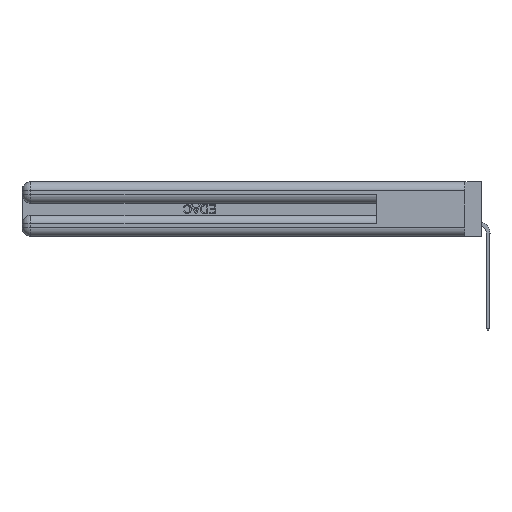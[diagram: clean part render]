
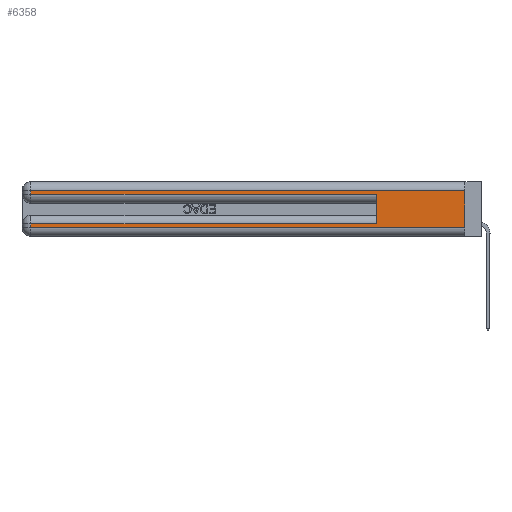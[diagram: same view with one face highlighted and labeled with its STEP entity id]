
A CAD part, left-side view. The second image highlights one B-rep face of the part: STEP entity #6358.
In plain terms, the highlighted planar face has unit normal (-1, 0, 0).
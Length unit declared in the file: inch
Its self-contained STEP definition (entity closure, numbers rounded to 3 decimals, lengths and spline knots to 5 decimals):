
#982 = ORIENTED_EDGE ( 'NONE', *, *, #1939, .T. ) ;
#1150 = CARTESIAN_POINT ( 'NONE',  ( 0., 0., 0.285 ) ) ;
#1248 = EDGE_CURVE ( 'NONE', #21710, #50398, #15956, .T. ) ;
#1607 = DIRECTION ( 'NONE',  ( 0., 0., 1. ) ) ;
#1939 = EDGE_CURVE ( 'NONE', #13976, #37767, #22024, .T. ) ;
#2253 = CARTESIAN_POINT ( 'NONE',  ( 0., 0., 0.37 ) ) ;
#3500 = ORIENTED_EDGE ( 'NONE', *, *, #37132, .T. ) ;
#4150 = VECTOR ( 'NONE', #22896, 39.37008 ) ;
#5775 = VECTOR ( 'NONE', #38353, 39.37008 ) ;
#6358 = ADVANCED_FACE ( 'NONE', ( #45294 ), #34544, .F. ) ;
#6715 = DIRECTION ( 'NONE',  ( 0., -1., 0. ) ) ;
#7668 = ORIENTED_EDGE ( 'NONE', *, *, #10380, .T. ) ;
#8444 = DIRECTION ( 'NONE',  ( 0., 1., 0. ) ) ;
#9440 = LINE ( 'NONE', #10826, #5775 ) ;
#9515 = CARTESIAN_POINT ( 'NONE',  ( 0., 2.94, 0.06 ) ) ;
#9645 = CARTESIAN_POINT ( 'NONE',  ( 0., 2.94, 0.37 ) ) ;
#10380 = EDGE_CURVE ( 'NONE', #46053, #13976, #9440, .T. ) ;
#10826 = CARTESIAN_POINT ( 'NONE',  ( 0., 2.94, 0.37 ) ) ;
#13364 = CARTESIAN_POINT ( 'NONE',  ( 0., 0.6, 0.145 ) ) ;
#13976 = VERTEX_POINT ( 'NONE', #9515 ) ;
#15003 = CARTESIAN_POINT ( 'NONE',  ( 0., 0., 0.085 ) ) ;
#15956 = LINE ( 'NONE', #13364, #32484 ) ;
#16480 = EDGE_CURVE ( 'NONE', #42474, #50621, #39028, .T. ) ;
#18364 = ORIENTED_EDGE ( 'NONE', *, *, #24891, .T. ) ;
#21710 = VERTEX_POINT ( 'NONE', #35023 ) ;
#22024 = LINE ( 'NONE', #45511, #50157 ) ;
#22172 = CARTESIAN_POINT ( 'NONE',  ( 0., 2.94, 0.085 ) ) ;
#22503 = LINE ( 'NONE', #15003, #4150 ) ;
#22896 = DIRECTION ( 'NONE',  ( 0., 1., 0. ) ) ;
#22976 = CARTESIAN_POINT ( 'NONE',  ( 0., 2.94, 0.285 ) ) ;
#24891 = EDGE_CURVE ( 'NONE', #31855, #50398, #48122, .T. ) ;
#26126 = DIRECTION ( 'NONE',  ( 0., 0., -1. ) ) ;
#26190 = ORIENTED_EDGE ( 'NONE', *, *, #38431, .T. ) ;
#27035 = LINE ( 'NONE', #2253, #39302 ) ;
#27101 = CARTESIAN_POINT ( 'NONE',  ( 0., 0., 0.06 ) ) ;
#29644 = VECTOR ( 'NONE', #32854, 39.37008 ) ;
#30046 = AXIS2_PLACEMENT_3D ( 'NONE', #38516, #38168, #45825 ) ;
#31814 = CARTESIAN_POINT ( 'NONE',  ( 0., 0., 0.31 ) ) ;
#31855 = VERTEX_POINT ( 'NONE', #22976 ) ;
#32065 = LINE ( 'NONE', #9645, #29644 ) ;
#32356 = CARTESIAN_POINT ( 'NONE',  ( 0., 2.94, 0.31 ) ) ;
#32364 = CARTESIAN_POINT ( 'NONE',  ( 0., 0., 0.31 ) ) ;
#32484 = VECTOR ( 'NONE', #1607, 39.37008 ) ;
#32854 = DIRECTION ( 'NONE',  ( 0., 0., -1. ) ) ;
#33517 = ORIENTED_EDGE ( 'NONE', *, *, #40971, .F. ) ;
#33825 = ORIENTED_EDGE ( 'NONE', *, *, #16480, .T. ) ;
#34544 = PLANE ( 'NONE',  #30046 ) ;
#35023 = CARTESIAN_POINT ( 'NONE',  ( 0., 0.6, 0.085 ) ) ;
#37132 = EDGE_CURVE ( 'NONE', #21710, #46053, #22503, .T. ) ;
#37767 = VERTEX_POINT ( 'NONE', #27101 ) ;
#37785 = VECTOR ( 'NONE', #40123, 39.37008 ) ;
#38168 = DIRECTION ( 'NONE',  ( 1., 0., 0. ) ) ;
#38353 = DIRECTION ( 'NONE',  ( 0., 0., -1. ) ) ;
#38431 = EDGE_CURVE ( 'NONE', #50621, #31855, #32065, .T. ) ;
#38516 = CARTESIAN_POINT ( 'NONE',  ( 0., 0., 0.37 ) ) ;
#39028 = LINE ( 'NONE', #31814, #48142 ) ;
#39302 = VECTOR ( 'NONE', #26126, 39.37008 ) ;
#40123 = DIRECTION ( 'NONE',  ( 0., -1., 0. ) ) ;
#40971 = EDGE_CURVE ( 'NONE', #42474, #37767, #27035, .T. ) ;
#42474 = VERTEX_POINT ( 'NONE', #32364 ) ;
#42952 = EDGE_LOOP ( 'NONE', ( #33517, #33825, #26190, #18364, #44401, #3500, #7668, #982 ) ) ;
#44401 = ORIENTED_EDGE ( 'NONE', *, *, #1248, .F. ) ;
#45294 = FACE_OUTER_BOUND ( 'NONE', #42952, .T. ) ;
#45511 = CARTESIAN_POINT ( 'NONE',  ( 0., 0., 0.06 ) ) ;
#45733 = CARTESIAN_POINT ( 'NONE',  ( 0., 0.6, 0.285 ) ) ;
#45825 = DIRECTION ( 'NONE',  ( 0., 0., -1. ) ) ;
#46053 = VERTEX_POINT ( 'NONE', #22172 ) ;
#48122 = LINE ( 'NONE', #1150, #37785 ) ;
#48142 = VECTOR ( 'NONE', #8444, 39.37008 ) ;
#50157 = VECTOR ( 'NONE', #6715, 39.37008 ) ;
#50398 = VERTEX_POINT ( 'NONE', #45733 ) ;
#50621 = VERTEX_POINT ( 'NONE', #32356 ) ;
